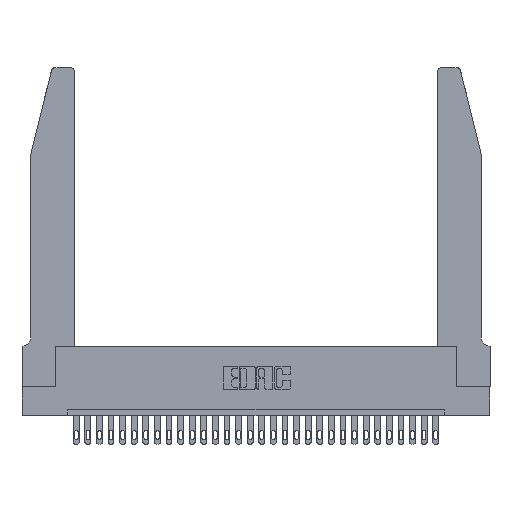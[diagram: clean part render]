
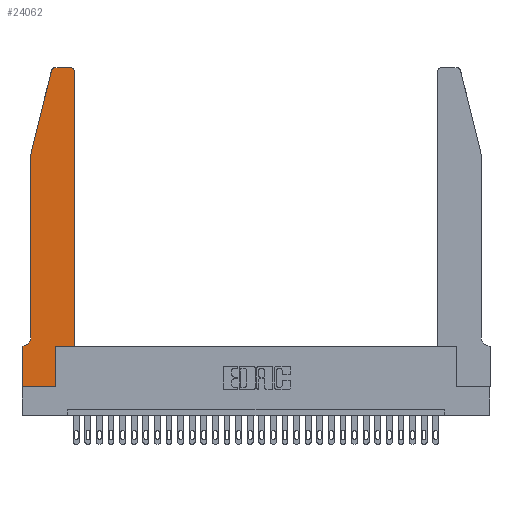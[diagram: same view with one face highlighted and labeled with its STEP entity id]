
A CAD part, top view. The second image highlights one B-rep face of the part: STEP entity #24062.
In plain terms, the highlighted planar face has unit normal (0, 0, 1).
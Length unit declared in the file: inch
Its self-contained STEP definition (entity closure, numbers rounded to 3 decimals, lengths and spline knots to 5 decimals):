
#16 = DIRECTION ( 'NONE',  ( -1., 0., 0. ) ) ;
#568 = CARTESIAN_POINT ( 'NONE',  ( 0.2865, 0.35, 0.37 ) ) ;
#727 = AXIS2_PLACEMENT_3D ( 'NONE', #15548, #3992, #3888 ) ;
#1192 = DIRECTION ( 'NONE',  ( 0., 0., 1. ) ) ;
#1613 = CARTESIAN_POINT ( 'NONE',  ( 0.0755, 2., 0.37 ) ) ;
#2185 = DIRECTION ( 'NONE',  ( 1., 0., 0. ) ) ;
#2251 = EDGE_CURVE ( 'NONE', #19301, #5044, #18993, .T. ) ;
#2497 = CARTESIAN_POINT ( 'NONE',  ( 0.4505, 0.35, 0.37 ) ) ;
#2945 = ORIENTED_EDGE ( 'NONE', *, *, #17845, .T. ) ;
#3607 = ORIENTED_EDGE ( 'NONE', *, *, #25026, .T. ) ;
#3652 = DIRECTION ( 'NONE',  ( 1., 0., 0. ) ) ;
#3888 = DIRECTION ( 'NONE',  ( 1., 0., 0. ) ) ;
#3992 = DIRECTION ( 'NONE',  ( 0., 0., 1. ) ) ;
#4146 = DIRECTION ( 'NONE',  ( 0., 1., 0. ) ) ;
#4190 = VERTEX_POINT ( 'NONE', #12595 ) ;
#4447 = EDGE_CURVE ( 'NONE', #5342, #4190, #15735, .T. ) ;
#5009 = VERTEX_POINT ( 'NONE', #19725 ) ;
#5044 = VERTEX_POINT ( 'NONE', #10822 ) ;
#5342 = VERTEX_POINT ( 'NONE', #2497 ) ;
#5706 = CARTESIAN_POINT ( 'NONE',  ( 0.2865, 0.35, 0.37 ) ) ;
#6079 = DIRECTION ( 'NONE',  ( -1., 0., 0. ) ) ;
#6742 = CARTESIAN_POINT ( 'NONE',  ( 0.284, 2.75, 0.37 ) ) ;
#6932 = EDGE_CURVE ( 'NONE', #14315, #28266, #7480, .T. ) ;
#7057 = VECTOR ( 'NONE', #4146, 39.37008 ) ;
#7200 = AXIS2_PLACEMENT_3D ( 'NONE', #10738, #29428, #17909 ) ;
#7428 = VECTOR ( 'NONE', #14304, 39.37008 ) ;
#7480 = LINE ( 'NONE', #20819, #24722 ) ;
#7748 = FACE_OUTER_BOUND ( 'NONE', #25217, .T. ) ;
#8039 = EDGE_CURVE ( 'NONE', #5009, #21637, #19168, .T. ) ;
#8061 = DIRECTION ( 'NONE',  ( 1., 0., 0. ) ) ;
#9168 = CIRCLE ( 'NONE', #15264, 0.03 ) ;
#9454 = CARTESIAN_POINT ( 'NONE',  ( 0.0755, 2., 0.37 ) ) ;
#9535 = LINE ( 'NONE', #10108, #24060 ) ;
#9878 = CARTESIAN_POINT ( 'NONE',  ( 0., 0., 0.37 ) ) ;
#10108 = CARTESIAN_POINT ( 'NONE',  ( 0.4505, 0.35, 0.37 ) ) ;
#10192 = DIRECTION ( 'NONE',  ( 0., 0., 1. ) ) ;
#10738 = CARTESIAN_POINT ( 'NONE',  ( 0.0055, 0.42, 0.37 ) ) ;
#10822 = CARTESIAN_POINT ( 'NONE',  ( 0.2865, 0., 0.37 ) ) ;
#12595 = CARTESIAN_POINT ( 'NONE',  ( 0.4505, 2.72, 0.37 ) ) ;
#13489 = CARTESIAN_POINT ( 'NONE',  ( 0.0755, 0.35, 0.37 ) ) ;
#13606 = LINE ( 'NONE', #9454, #7428 ) ;
#13660 = CARTESIAN_POINT ( 'NONE',  ( 0., 0., 0.37 ) ) ;
#13802 = CARTESIAN_POINT ( 'NONE',  ( 0.0755, 2., 0.37 ) ) ;
#14304 = DIRECTION ( 'NONE',  ( -0.239, -0.971, 0. ) ) ;
#14315 = VERTEX_POINT ( 'NONE', #29438 ) ;
#14929 = CARTESIAN_POINT ( 'NONE',  ( 0., 0., 0.37 ) ) ;
#15264 = AXIS2_PLACEMENT_3D ( 'NONE', #19596, #10192, #22144 ) ;
#15514 = VERTEX_POINT ( 'NONE', #23695 ) ;
#15548 = CARTESIAN_POINT ( 'NONE',  ( 0.284, 2.72, 0.37 ) ) ;
#15735 = LINE ( 'NONE', #27207, #7057 ) ;
#15852 = EDGE_CURVE ( 'NONE', #28266, #18947, #16916, .T. ) ;
#16000 = ORIENTED_EDGE ( 'NONE', *, *, #15852, .T. ) ;
#16864 = VERTEX_POINT ( 'NONE', #568 ) ;
#16916 = CIRCLE ( 'NONE', #727, 0.03 ) ;
#16959 = DIRECTION ( 'NONE',  ( 0., 1., 0. ) ) ;
#17007 = EDGE_CURVE ( 'NONE', #15514, #5009, #25993, .T. ) ;
#17200 = CARTESIAN_POINT ( 'NONE',  ( 0., 0.35, 0.37 ) ) ;
#17638 = DIRECTION ( 'NONE',  ( 0., -1., 0. ) ) ;
#17780 = ORIENTED_EDGE ( 'NONE', *, *, #19341, .T. ) ;
#17845 = EDGE_CURVE ( 'NONE', #18947, #27572, #13606, .T. ) ;
#17909 = DIRECTION ( 'NONE',  ( -1., 0., 0. ) ) ;
#18180 = LINE ( 'NONE', #14929, #26576 ) ;
#18721 = EDGE_CURVE ( 'NONE', #16864, #5342, #9535, .T. ) ;
#18775 = ORIENTED_EDGE ( 'NONE', *, *, #22564, .T. ) ;
#18947 = VERTEX_POINT ( 'NONE', #22863 ) ;
#18993 = LINE ( 'NONE', #13660, #29925 ) ;
#19168 = LINE ( 'NONE', #13489, #23897 ) ;
#19301 = VERTEX_POINT ( 'NONE', #9878 ) ;
#19341 = EDGE_CURVE ( 'NONE', #21637, #19301, #18180, .T. ) ;
#19596 = CARTESIAN_POINT ( 'NONE',  ( 0.4205, 2.72, 0.37 ) ) ;
#19725 = CARTESIAN_POINT ( 'NONE',  ( 0.0055, 0.35, 0.37 ) ) ;
#20819 = CARTESIAN_POINT ( 'NONE',  ( 0.2605, 2.75, 0.37 ) ) ;
#21033 = EDGE_CURVE ( 'NONE', #27572, #15514, #27533, .T. ) ;
#21637 = VERTEX_POINT ( 'NONE', #17200 ) ;
#22144 = DIRECTION ( 'NONE',  ( 1., 0., 0. ) ) ;
#22241 = ORIENTED_EDGE ( 'NONE', *, *, #2251, .T. ) ;
#22564 = EDGE_CURVE ( 'NONE', #5044, #16864, #23462, .T. ) ;
#22863 = CARTESIAN_POINT ( 'NONE',  ( 0.25487, 2.72718, 0.37 ) ) ;
#22904 = ORIENTED_EDGE ( 'NONE', *, *, #4447, .T. ) ;
#23158 = ORIENTED_EDGE ( 'NONE', *, *, #17007, .T. ) ;
#23462 = LINE ( 'NONE', #5706, #25287 ) ;
#23695 = CARTESIAN_POINT ( 'NONE',  ( 0.0755, 0.42, 0.37 ) ) ;
#23897 = VECTOR ( 'NONE', #6079, 39.37008 ) ;
#24060 = VECTOR ( 'NONE', #8061, 39.37008 ) ;
#24062 = ADVANCED_FACE ( 'NONE', ( #7748 ), #26908, .T. ) ;
#24722 = VECTOR ( 'NONE', #16, 39.37008 ) ;
#24957 = ORIENTED_EDGE ( 'NONE', *, *, #18721, .T. ) ;
#25026 = EDGE_CURVE ( 'NONE', #4190, #14315, #9168, .T. ) ;
#25217 = EDGE_LOOP ( 'NONE', ( #26803, #16000, #2945, #28912, #23158, #29568, #17780, #22241, #18775, #24957, #22904, #3607 ) ) ;
#25287 = VECTOR ( 'NONE', #16959, 39.37008 ) ;
#25993 = CIRCLE ( 'NONE', #7200, 0.07 ) ;
#26531 = DIRECTION ( 'NONE',  ( 0., -1., 0. ) ) ;
#26576 = VECTOR ( 'NONE', #26531, 39.37008 ) ;
#26700 = CARTESIAN_POINT ( 'NONE',  ( 0., 0.35, 0.37 ) ) ;
#26803 = ORIENTED_EDGE ( 'NONE', *, *, #6932, .T. ) ;
#26908 = PLANE ( 'NONE',  #27336 ) ;
#27207 = CARTESIAN_POINT ( 'NONE',  ( 0.4505, 0.35, 0.37 ) ) ;
#27336 = AXIS2_PLACEMENT_3D ( 'NONE', #26700, #1192, #3652 ) ;
#27533 = LINE ( 'NONE', #1613, #28253 ) ;
#27572 = VERTEX_POINT ( 'NONE', #13802 ) ;
#28253 = VECTOR ( 'NONE', #17638, 39.37008 ) ;
#28266 = VERTEX_POINT ( 'NONE', #6742 ) ;
#28912 = ORIENTED_EDGE ( 'NONE', *, *, #21033, .T. ) ;
#29428 = DIRECTION ( 'NONE',  ( 0., 0., -1. ) ) ;
#29438 = CARTESIAN_POINT ( 'NONE',  ( 0.4205, 2.75, 0.37 ) ) ;
#29568 = ORIENTED_EDGE ( 'NONE', *, *, #8039, .T. ) ;
#29925 = VECTOR ( 'NONE', #2185, 39.37008 ) ;
